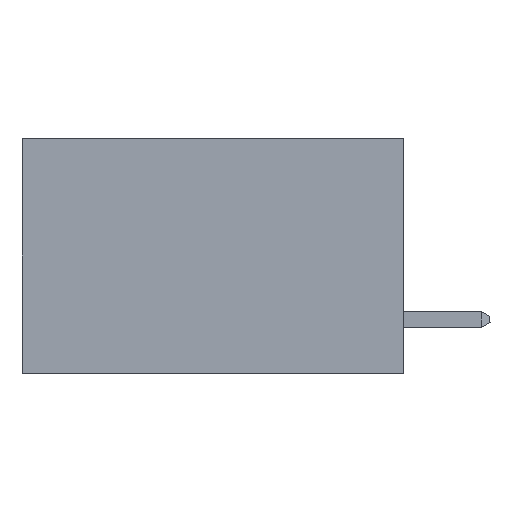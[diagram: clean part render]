
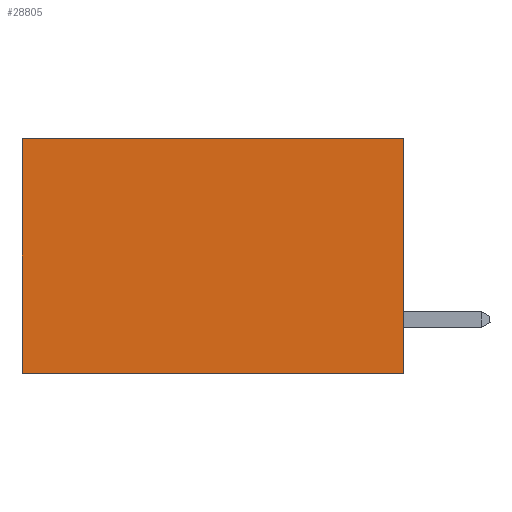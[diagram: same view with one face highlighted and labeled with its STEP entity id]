
A CAD part, left-side view. The second image highlights one B-rep face of the part: STEP entity #28805.
In plain terms, the highlighted planar face has unit normal (-1, 0, 0).
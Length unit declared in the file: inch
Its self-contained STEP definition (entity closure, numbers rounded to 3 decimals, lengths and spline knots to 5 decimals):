
#65 = ORIENTED_EDGE ( 'NONE', *, *, #1274, .F. ) ;
#787 = VERTEX_POINT ( 'NONE', #23846 ) ;
#790 = VECTOR ( 'NONE', #39494, 39.37008 ) ;
#1274 = EDGE_CURVE ( 'NONE', #25733, #36309, #25147, .T. ) ;
#5054 = DIRECTION ( 'NONE',  ( 0., 1., 0. ) ) ;
#6358 = LINE ( 'NONE', #11069, #790 ) ;
#7925 = ORIENTED_EDGE ( 'NONE', *, *, #39636, .F. ) ;
#8309 = ORIENTED_EDGE ( 'NONE', *, *, #14039, .T. ) ;
#8420 = VERTEX_POINT ( 'NONE', #17062 ) ;
#8667 = EDGE_LOOP ( 'NONE', ( #43411, #65, #7925, #8309 ) ) ;
#9202 = PLANE ( 'NONE',  #9863 ) ;
#9863 = AXIS2_PLACEMENT_3D ( 'NONE', #27077, #10269, #45882 ) ;
#10269 = DIRECTION ( 'NONE',  ( 1., 0., 0. ) ) ;
#10599 = VECTOR ( 'NONE', #32702, 39.37008 ) ;
#10995 = CARTESIAN_POINT ( 'NONE',  ( 0.2875, 0.6, 0. ) ) ;
#11069 = CARTESIAN_POINT ( 'NONE',  ( 0.2875, 0., 0. ) ) ;
#11393 = CARTESIAN_POINT ( 'NONE',  ( 0.2875, 0., -0.37 ) ) ;
#12715 = FACE_OUTER_BOUND ( 'NONE', #8667, .T. ) ;
#14039 = EDGE_CURVE ( 'NONE', #787, #8420, #22859, .T. ) ;
#16053 = VECTOR ( 'NONE', #25276, 39.37008 ) ;
#17062 = CARTESIAN_POINT ( 'NONE',  ( 0.2875, 0.6, 0. ) ) ;
#19588 = CARTESIAN_POINT ( 'NONE',  ( 0.2875, 0., -0.37 ) ) ;
#19783 = CARTESIAN_POINT ( 'NONE',  ( 0.2875, 0.6, -0.37 ) ) ;
#20748 = CARTESIAN_POINT ( 'NONE',  ( 0.2875, 0., 0. ) ) ;
#21816 = VECTOR ( 'NONE', #5054, 39.37008 ) ;
#22859 = LINE ( 'NONE', #20748, #10599 ) ;
#23846 = CARTESIAN_POINT ( 'NONE',  ( 0.2875, 0., 0. ) ) ;
#25147 = LINE ( 'NONE', #11393, #21816 ) ;
#25276 = DIRECTION ( 'NONE',  ( 0., 0., -1. ) ) ;
#25733 = VERTEX_POINT ( 'NONE', #19588 ) ;
#27077 = CARTESIAN_POINT ( 'NONE',  ( 0.2875, 0., 0. ) ) ;
#28805 = ADVANCED_FACE ( 'NONE', ( #12715 ), #9202, .F. ) ;
#32189 = EDGE_CURVE ( 'NONE', #8420, #36309, #36744, .T. ) ;
#32702 = DIRECTION ( 'NONE',  ( 0., 1., 0. ) ) ;
#36309 = VERTEX_POINT ( 'NONE', #19783 ) ;
#36744 = LINE ( 'NONE', #10995, #16053 ) ;
#39494 = DIRECTION ( 'NONE',  ( 0., 0., -1. ) ) ;
#39636 = EDGE_CURVE ( 'NONE', #787, #25733, #6358, .T. ) ;
#43411 = ORIENTED_EDGE ( 'NONE', *, *, #32189, .T. ) ;
#45882 = DIRECTION ( 'NONE',  ( 0., 0., -1. ) ) ;
